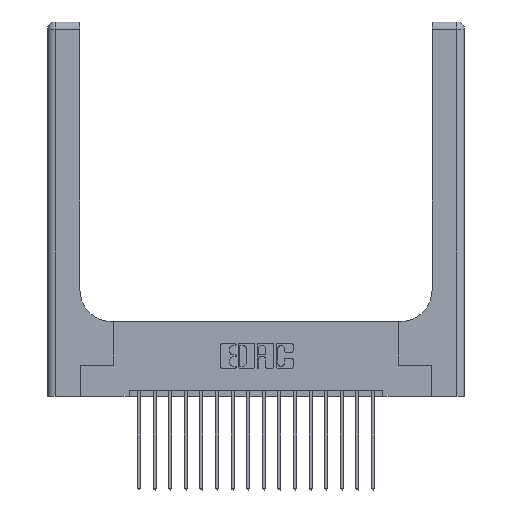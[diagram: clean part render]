
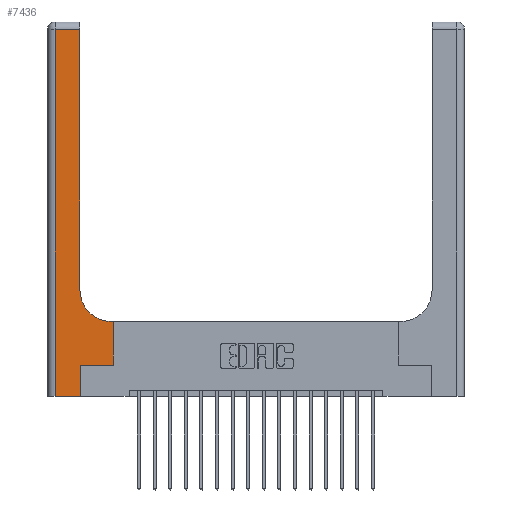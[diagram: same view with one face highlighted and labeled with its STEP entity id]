
A CAD part, top view. The second image highlights one B-rep face of the part: STEP entity #7436.
In plain terms, the highlighted planar face has unit normal (0, 0, 1).
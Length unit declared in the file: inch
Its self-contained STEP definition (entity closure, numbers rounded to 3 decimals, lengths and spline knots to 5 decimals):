
#74 = CARTESIAN_POINT ( 'NONE',  ( 0.528, 0.6, 0.37 ) ) ;
#75 = EDGE_CURVE ( 'NONE', #16817, #14901, #2244, .T. ) ;
#484 = CARTESIAN_POINT ( 'NONE',  ( 0.26, 3., 0.37 ) ) ;
#586 = EDGE_CURVE ( 'NONE', #1994, #2993, #1121, .T. ) ;
#702 = VECTOR ( 'NONE', #4878, 39.37008 ) ;
#1121 = LINE ( 'NONE', #8959, #18607 ) ;
#1730 = ORIENTED_EDGE ( 'NONE', *, *, #5185, .T. ) ;
#1736 = LINE ( 'NONE', #13523, #1903 ) ;
#1749 = LINE ( 'NONE', #13834, #16141 ) ;
#1903 = VECTOR ( 'NONE', #4513, 39.37008 ) ;
#1964 = AXIS2_PLACEMENT_3D ( 'NONE', #16495, #2850, #8902 ) ;
#1974 = AXIS2_PLACEMENT_3D ( 'NONE', #3752, #2073, #3462 ) ;
#1994 = VERTEX_POINT ( 'NONE', #6252 ) ;
#2073 = DIRECTION ( 'NONE',  ( 0., 0., -1. ) ) ;
#2104 = EDGE_CURVE ( 'NONE', #14901, #18391, #13678, .T. ) ;
#2170 = CARTESIAN_POINT ( 'NONE',  ( 0.26, 0.85, 0.37 ) ) ;
#2244 = LINE ( 'NONE', #6899, #16976 ) ;
#2850 = DIRECTION ( 'NONE',  ( 0., 0., -1. ) ) ;
#2872 = VECTOR ( 'NONE', #16295, 39.37008 ) ;
#2993 = VERTEX_POINT ( 'NONE', #12928 ) ;
#3384 = EDGE_CURVE ( 'NONE', #18391, #18070, #14053, .T. ) ;
#3462 = DIRECTION ( 'NONE',  ( 1., 0., 0. ) ) ;
#3491 = CARTESIAN_POINT ( 'NONE',  ( 0., 2.94, 0.37 ) ) ;
#3752 = CARTESIAN_POINT ( 'NONE',  ( 0.51, 0.85, 0.37 ) ) ;
#4091 = ORIENTED_EDGE ( 'NONE', *, *, #586, .T. ) ;
#4513 = DIRECTION ( 'NONE',  ( 1., 0., 0. ) ) ;
#4861 = ORIENTED_EDGE ( 'NONE', *, *, #18974, .T. ) ;
#4878 = DIRECTION ( 'NONE',  ( -1., 0., 0. ) ) ;
#5126 = VERTEX_POINT ( 'NONE', #11329 ) ;
#5185 = EDGE_CURVE ( 'NONE', #18070, #5126, #14275, .T. ) ;
#5217 = VERTEX_POINT ( 'NONE', #9546 ) ;
#5919 = FACE_OUTER_BOUND ( 'NONE', #12172, .T. ) ;
#6252 = CARTESIAN_POINT ( 'NONE',  ( 0.265, 0.25, 0.37 ) ) ;
#6543 = DIRECTION ( 'NONE',  ( 0., 1., 0. ) ) ;
#6555 = VECTOR ( 'NONE', #6543, 39.37008 ) ;
#6899 = CARTESIAN_POINT ( 'NONE',  ( 0.26, 0.6, 0.37 ) ) ;
#7333 = EDGE_CURVE ( 'NONE', #5126, #17817, #10294, .T. ) ;
#7436 = ADVANCED_FACE ( 'NONE', ( #5919 ), #16394, .F. ) ;
#7531 = EDGE_CURVE ( 'NONE', #2993, #16817, #1749, .T. ) ;
#7902 = DIRECTION ( 'NONE',  ( 0., 1., 0. ) ) ;
#8902 = DIRECTION ( 'NONE',  ( -1., 0., 0. ) ) ;
#8959 = CARTESIAN_POINT ( 'NONE',  ( 0.265, 0.25, 0.37 ) ) ;
#9546 = CARTESIAN_POINT ( 'NONE',  ( 0.265, 0., 0.37 ) ) ;
#9615 = EDGE_CURVE ( 'NONE', #5217, #1994, #19508, .T. ) ;
#9712 = ORIENTED_EDGE ( 'NONE', *, *, #2104, .T. ) ;
#10060 = CARTESIAN_POINT ( 'NONE',  ( 0.51, 0.6, 0.37 ) ) ;
#10119 = ORIENTED_EDGE ( 'NONE', *, *, #9615, .T. ) ;
#10121 = CARTESIAN_POINT ( 'NONE',  ( 0.265, 0., 0.37 ) ) ;
#10294 = LINE ( 'NONE', #19097, #2872 ) ;
#10863 = CARTESIAN_POINT ( 'NONE',  ( 0.26, 2.94, 0.37 ) ) ;
#10961 = VECTOR ( 'NONE', #14854, 39.37008 ) ;
#11329 = CARTESIAN_POINT ( 'NONE',  ( 0.06, 2.94, 0.37 ) ) ;
#12172 = EDGE_LOOP ( 'NONE', ( #18262, #1730, #18624, #4861, #10119, #4091, #14826, #14055, #9712 ) ) ;
#12846 = DIRECTION ( 'NONE',  ( -1., 0., 0. ) ) ;
#12928 = CARTESIAN_POINT ( 'NONE',  ( 0.528, 0.25, 0.37 ) ) ;
#13523 = CARTESIAN_POINT ( 'NONE',  ( 0., 0., 0.37 ) ) ;
#13678 = CIRCLE ( 'NONE', #1974, 0.25 ) ;
#13834 = CARTESIAN_POINT ( 'NONE',  ( 0.528, 0.25, 0.37 ) ) ;
#14053 = LINE ( 'NONE', #484, #6555 ) ;
#14055 = ORIENTED_EDGE ( 'NONE', *, *, #75, .T. ) ;
#14275 = LINE ( 'NONE', #3491, #702 ) ;
#14826 = ORIENTED_EDGE ( 'NONE', *, *, #7531, .T. ) ;
#14854 = DIRECTION ( 'NONE',  ( 0., 1., 0. ) ) ;
#14901 = VERTEX_POINT ( 'NONE', #10060 ) ;
#16141 = VECTOR ( 'NONE', #7902, 39.37008 ) ;
#16295 = DIRECTION ( 'NONE',  ( 0., -1., 0. ) ) ;
#16394 = PLANE ( 'NONE',  #1964 ) ;
#16495 = CARTESIAN_POINT ( 'NONE',  ( 0., 3., 0.37 ) ) ;
#16817 = VERTEX_POINT ( 'NONE', #74 ) ;
#16976 = VECTOR ( 'NONE', #12846, 39.37008 ) ;
#17679 = CARTESIAN_POINT ( 'NONE',  ( 0.06, 0., 0.37 ) ) ;
#17817 = VERTEX_POINT ( 'NONE', #17679 ) ;
#17850 = DIRECTION ( 'NONE',  ( 1., 0., 0. ) ) ;
#18070 = VERTEX_POINT ( 'NONE', #10863 ) ;
#18262 = ORIENTED_EDGE ( 'NONE', *, *, #3384, .T. ) ;
#18391 = VERTEX_POINT ( 'NONE', #2170 ) ;
#18607 = VECTOR ( 'NONE', #17850, 39.37008 ) ;
#18624 = ORIENTED_EDGE ( 'NONE', *, *, #7333, .T. ) ;
#18974 = EDGE_CURVE ( 'NONE', #17817, #5217, #1736, .T. ) ;
#19097 = CARTESIAN_POINT ( 'NONE',  ( 0.06, 3., 0.37 ) ) ;
#19508 = LINE ( 'NONE', #10121, #10961 ) ;
